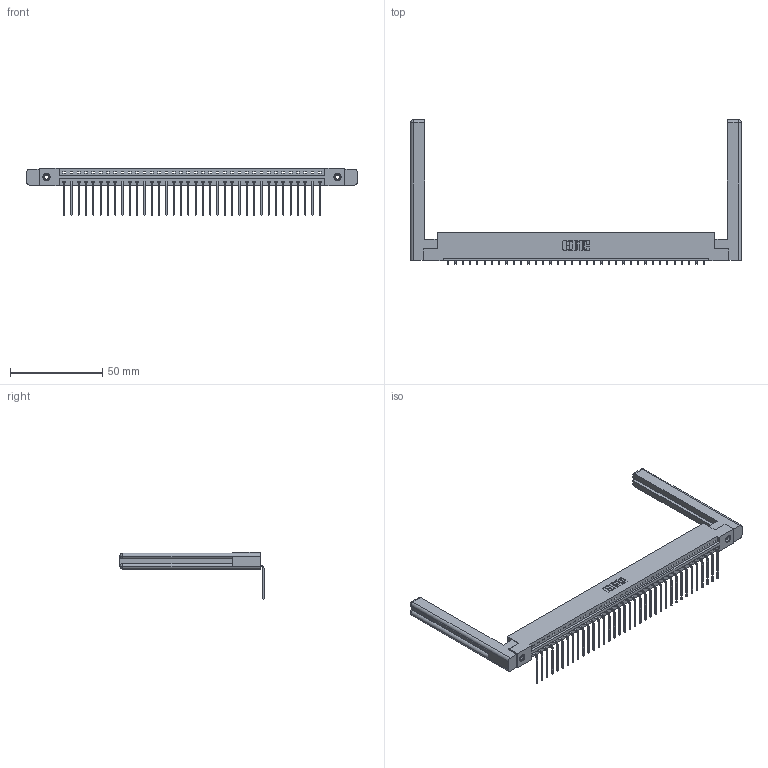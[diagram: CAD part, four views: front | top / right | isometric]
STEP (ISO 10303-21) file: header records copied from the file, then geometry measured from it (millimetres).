
FILE_DESCRIPTION (( 'STEP AP203' ), '1' );
FILE_NAME ('387-036-559-158.STEP', '2019-10-04T13:55:54', ( '' ), ( '' ), 'SwSTEP 2.0', 'SolidWorks 2016', '' );
FILE_SCHEMA (( 'CONFIG_CONTROL_DESIGN' ));
Length unit declared in the file: inch
Products named in the file (5): 387-036-559-158; 345-250-001_345-250-001-102; 307-220-058; 337 Part_Flush Mounting Lugs - 0.156 Dia-TI; 345-292-001_558 559 Tail - 1
Assembly tree (41 placements, depth 2):
  387-036-559-158
    337 Part_Flush Mounting Lugs - 0.156 Dia-TI
    345-292-001_558 559 Tail - 1  x36
    345-250-001_345-250-001-102  x2
    307-220-058  x2
Bounding box: 179.27 x 78.17 x 25.53 mm (x, y, z)
Volume: 25839.5 mm3; surface area: 25216.8 mm2
Topology: 41 solids, 41 shells, 2560 faces, 7649 edges, 5038 vertices
Faces by surface type: plane 1882, cylinder 654, cone 12, torus 12
Entity records: 30254 total; most frequent: CARTESIAN_POINT 5269, ORIENTED_EDGE 5180, DIRECTION 4466, EDGE_CURVE 2590, VECTOR 2414, LINE 2414, VERTEX_POINT 1718, AXIS2_PLACEMENT_3D 1026
